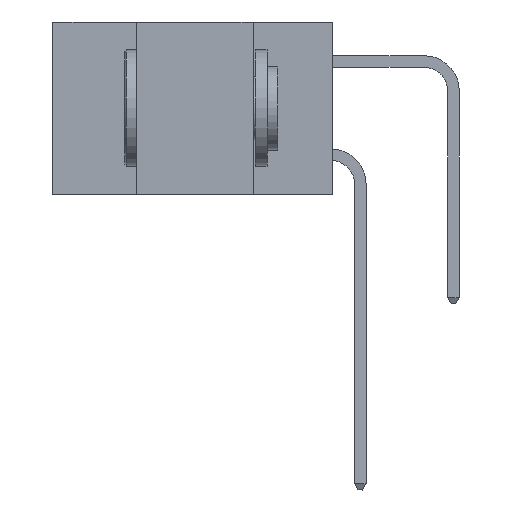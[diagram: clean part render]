
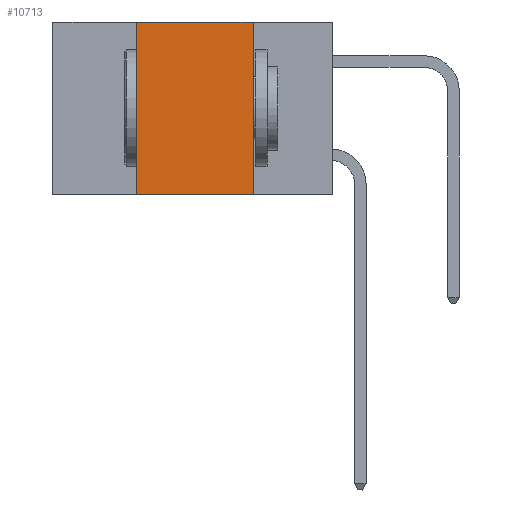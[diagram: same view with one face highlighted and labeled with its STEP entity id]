
A CAD part, left-side view. The second image highlights one B-rep face of the part: STEP entity #10713.
In plain terms, the highlighted planar face has unit normal (-1, 0, 0).
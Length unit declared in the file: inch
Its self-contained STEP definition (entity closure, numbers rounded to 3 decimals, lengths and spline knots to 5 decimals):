
#319 = VECTOR ( 'NONE', #10740, 39.37008 ) ;
#603 = CARTESIAN_POINT ( 'NONE',  ( 0., 0.6, 0. ) ) ;
#799 = ORIENTED_EDGE ( 'NONE', *, *, #4759, .F. ) ;
#1608 = LINE ( 'NONE', #1810, #5579 ) ;
#1810 = CARTESIAN_POINT ( 'NONE',  ( 0., 0.6, -0.37 ) ) ;
#1946 = CARTESIAN_POINT ( 'NONE',  ( 0., 0.42, 0. ) ) ;
#2295 = EDGE_CURVE ( 'NONE', #6252, #4510, #2773, .T. ) ;
#2504 = VERTEX_POINT ( 'NONE', #4681 ) ;
#2773 = LINE ( 'NONE', #6154, #9250 ) ;
#2839 = ORIENTED_EDGE ( 'NONE', *, *, #2295, .F. ) ;
#2974 = CARTESIAN_POINT ( 'NONE',  ( 0., 0.42, -0.37 ) ) ;
#3039 = PLANE ( 'NONE',  #9480 ) ;
#3153 = DIRECTION ( 'NONE',  ( 0., 0., -1. ) ) ;
#3194 = CARTESIAN_POINT ( 'NONE',  ( 0., 0.17, -0.37 ) ) ;
#3286 = ORIENTED_EDGE ( 'NONE', *, *, #5796, .T. ) ;
#3415 = VERTEX_POINT ( 'NONE', #2974 ) ;
#4510 = VERTEX_POINT ( 'NONE', #4741 ) ;
#4570 = EDGE_CURVE ( 'NONE', #3415, #6252, #5641, .T. ) ;
#4681 = CARTESIAN_POINT ( 'NONE',  ( 0., 0.17, -0.37 ) ) ;
#4741 = CARTESIAN_POINT ( 'NONE',  ( 0., 0.17, 0. ) ) ;
#4759 = EDGE_CURVE ( 'NONE', #4510, #2504, #9140, .T. ) ;
#5265 = DIRECTION ( 'NONE',  ( 0., -1., 0. ) ) ;
#5579 = VECTOR ( 'NONE', #5265, 39.37008 ) ;
#5641 = LINE ( 'NONE', #8056, #319 ) ;
#5654 = FACE_OUTER_BOUND ( 'NONE', #6838, .T. ) ;
#5796 = EDGE_CURVE ( 'NONE', #3415, #2504, #1608, .T. ) ;
#6154 = CARTESIAN_POINT ( 'NONE',  ( 0., 0.6, 0. ) ) ;
#6252 = VERTEX_POINT ( 'NONE', #1946 ) ;
#6838 = EDGE_LOOP ( 'NONE', ( #799, #2839, #9387, #3286 ) ) ;
#7722 = VECTOR ( 'NONE', #10909, 39.37008 ) ;
#7899 = DIRECTION ( 'NONE',  ( 0., -1., 0. ) ) ;
#8056 = CARTESIAN_POINT ( 'NONE',  ( 0., 0.42, -0.37 ) ) ;
#9140 = LINE ( 'NONE', #3194, #7722 ) ;
#9250 = VECTOR ( 'NONE', #7899, 39.37008 ) ;
#9387 = ORIENTED_EDGE ( 'NONE', *, *, #4570, .F. ) ;
#9480 = AXIS2_PLACEMENT_3D ( 'NONE', #603, #10304, #3153 ) ;
#10304 = DIRECTION ( 'NONE',  ( 1., 0., 0. ) ) ;
#10713 = ADVANCED_FACE ( 'NONE', ( #5654 ), #3039, .F. ) ;
#10740 = DIRECTION ( 'NONE',  ( 0., 0., 1. ) ) ;
#10909 = DIRECTION ( 'NONE',  ( 0., 0., -1. ) ) ;
